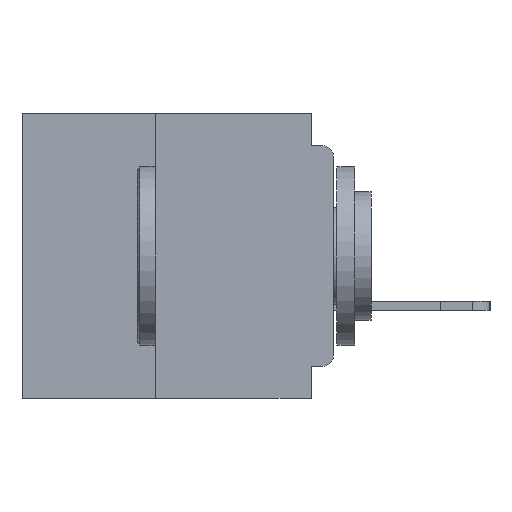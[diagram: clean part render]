
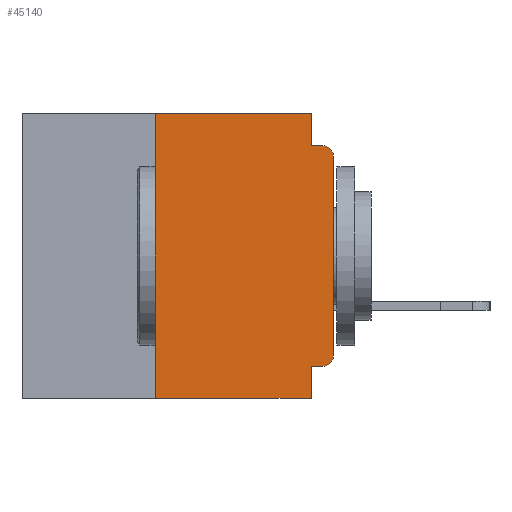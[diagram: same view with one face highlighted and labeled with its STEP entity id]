
A CAD part, left-side view. The second image highlights one B-rep face of the part: STEP entity #45140.
In plain terms, the highlighted planar face has unit normal (-1, 0, 0).
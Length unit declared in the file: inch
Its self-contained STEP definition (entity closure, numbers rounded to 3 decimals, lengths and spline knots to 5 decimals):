
#1364 = VECTOR ( 'NONE', #36220, 39.37008 ) ;
#1433 = VERTEX_POINT ( 'NONE', #27014 ) ;
#1634 = VECTOR ( 'NONE', #19848, 39.37008 ) ;
#1896 = VERTEX_POINT ( 'NONE', #3787 ) ;
#2962 = ORIENTED_EDGE ( 'NONE', *, *, #20656, .T. ) ;
#3313 = VERTEX_POINT ( 'NONE', #28480 ) ;
#3325 = FACE_OUTER_BOUND ( 'NONE', #16595, .T. ) ;
#3534 = DIRECTION ( 'NONE',  ( 0., -1., 0. ) ) ;
#3787 = CARTESIAN_POINT ( 'NONE',  ( 0., 0.031, -0.4 ) ) ;
#5828 = EDGE_CURVE ( 'NONE', #42242, #43689, #36878, .T. ) ;
#5871 = CARTESIAN_POINT ( 'NONE',  ( 0., 0.437, 0. ) ) ;
#6412 = LINE ( 'NONE', #35386, #26719 ) ;
#7238 = CARTESIAN_POINT ( 'NONE',  ( 0., 0.015, -0.06 ) ) ;
#7446 = ORIENTED_EDGE ( 'NONE', *, *, #46930, .F. ) ;
#8452 = AXIS2_PLACEMENT_3D ( 'NONE', #19461, #46099, #23297 ) ;
#9111 = CIRCLE ( 'NONE', #8452, 0.015 ) ;
#9118 = EDGE_CURVE ( 'NONE', #3313, #1896, #33009, .T. ) ;
#9823 = CARTESIAN_POINT ( 'NONE',  ( 0., 0., -0.355 ) ) ;
#10975 = AXIS2_PLACEMENT_3D ( 'NONE', #36495, #21384, #48017 ) ;
#11075 = DIRECTION ( 'NONE',  ( 0., 0., -1. ) ) ;
#12781 = CARTESIAN_POINT ( 'NONE',  ( 0., 0.25, -0.4 ) ) ;
#13275 = ORIENTED_EDGE ( 'NONE', *, *, #5828, .F. ) ;
#14366 = ORIENTED_EDGE ( 'NONE', *, *, #28256, .F. ) ;
#14756 = VERTEX_POINT ( 'NONE', #32859 ) ;
#15012 = CARTESIAN_POINT ( 'NONE',  ( 0., 0.25, 0. ) ) ;
#15478 = ORIENTED_EDGE ( 'NONE', *, *, #43362, .F. ) ;
#16577 = CARTESIAN_POINT ( 'NONE',  ( 0., 0.437, -0.4 ) ) ;
#16595 = EDGE_LOOP ( 'NONE', ( #2962, #45476, #13275, #15478, #44065, #14366, #34073, #23462, #7446, #43950 ) ) ;
#16642 = DIRECTION ( 'NONE',  ( 0., 0., 1. ) ) ;
#17417 = VERTEX_POINT ( 'NONE', #36059 ) ;
#19124 = LINE ( 'NONE', #9823, #39336 ) ;
#19386 = LINE ( 'NONE', #12781, #38417 ) ;
#19461 = CARTESIAN_POINT ( 'NONE',  ( 0., 0.015, -0.34 ) ) ;
#19848 = DIRECTION ( 'NONE',  ( 0., 0., 1. ) ) ;
#20656 = EDGE_CURVE ( 'NONE', #30267, #1433, #42254, .T. ) ;
#21384 = DIRECTION ( 'NONE',  ( 1., 0., 0. ) ) ;
#22906 = CIRCLE ( 'NONE', #28927, 0.015 ) ;
#23297 = DIRECTION ( 'NONE',  ( 0., 0., -1. ) ) ;
#23462 = ORIENTED_EDGE ( 'NONE', *, *, #47915, .F. ) ;
#24372 = VECTOR ( 'NONE', #29343, 39.37008 ) ;
#25028 = PLANE ( 'NONE',  #10975 ) ;
#25037 = DIRECTION ( 'NONE',  ( 0., 1., 0. ) ) ;
#26719 = VECTOR ( 'NONE', #46736, 39.37008 ) ;
#26741 = VECTOR ( 'NONE', #3534, 39.37008 ) ;
#27014 = CARTESIAN_POINT ( 'NONE',  ( 0., 0., -0.06 ) ) ;
#28256 = EDGE_CURVE ( 'NONE', #3313, #44262, #19386, .T. ) ;
#28480 = CARTESIAN_POINT ( 'NONE',  ( 0., 0.25, -0.4 ) ) ;
#28710 = EDGE_CURVE ( 'NONE', #17417, #30267, #9111, .T. ) ;
#28927 = AXIS2_PLACEMENT_3D ( 'NONE', #7238, #33923, #11075 ) ;
#29343 = DIRECTION ( 'NONE',  ( 0., 0., -1. ) ) ;
#29833 = CARTESIAN_POINT ( 'NONE',  ( 0., 0.015, -0.045 ) ) ;
#30267 = VERTEX_POINT ( 'NONE', #33753 ) ;
#31727 = DIRECTION ( 'NONE',  ( 0., -1., 0. ) ) ;
#32859 = CARTESIAN_POINT ( 'NONE',  ( 0., 0.031, -0.355 ) ) ;
#33009 = LINE ( 'NONE', #16577, #44384 ) ;
#33212 = CARTESIAN_POINT ( 'NONE',  ( 0., 0.031, 0. ) ) ;
#33753 = CARTESIAN_POINT ( 'NONE',  ( 0., 0., -0.34 ) ) ;
#33923 = DIRECTION ( 'NONE',  ( -1., 0., 0. ) ) ;
#34073 = ORIENTED_EDGE ( 'NONE', *, *, #9118, .T. ) ;
#35386 = CARTESIAN_POINT ( 'NONE',  ( 0., 0.031, 0. ) ) ;
#36059 = CARTESIAN_POINT ( 'NONE',  ( 0., 0.015, -0.355 ) ) ;
#36220 = DIRECTION ( 'NONE',  ( 0., -1., 0. ) ) ;
#36495 = CARTESIAN_POINT ( 'NONE',  ( 0., 0.437, 0. ) ) ;
#36734 = VERTEX_POINT ( 'NONE', #33212 ) ;
#36878 = LINE ( 'NONE', #49217, #26741 ) ;
#38056 = EDGE_CURVE ( 'NONE', #1433, #43689, #22906, .T. ) ;
#38417 = VECTOR ( 'NONE', #16642, 39.37008 ) ;
#38803 = CARTESIAN_POINT ( 'NONE',  ( 0., 0., 0. ) ) ;
#39336 = VECTOR ( 'NONE', #25037, 39.37008 ) ;
#39982 = CARTESIAN_POINT ( 'NONE',  ( 0., 0.031, -0.045 ) ) ;
#40212 = EDGE_CURVE ( 'NONE', #44262, #36734, #41994, .T. ) ;
#40858 = CARTESIAN_POINT ( 'NONE',  ( 0., 0.031, -0.4 ) ) ;
#41994 = LINE ( 'NONE', #5871, #1364 ) ;
#42242 = VERTEX_POINT ( 'NONE', #39982 ) ;
#42254 = LINE ( 'NONE', #38803, #1634 ) ;
#43362 = EDGE_CURVE ( 'NONE', #36734, #42242, #6412, .T. ) ;
#43689 = VERTEX_POINT ( 'NONE', #29833 ) ;
#43950 = ORIENTED_EDGE ( 'NONE', *, *, #28710, .T. ) ;
#44065 = ORIENTED_EDGE ( 'NONE', *, *, #40212, .F. ) ;
#44262 = VERTEX_POINT ( 'NONE', #15012 ) ;
#44384 = VECTOR ( 'NONE', #31727, 39.37008 ) ;
#45140 = ADVANCED_FACE ( 'NONE', ( #3325 ), #25028, .F. ) ;
#45476 = ORIENTED_EDGE ( 'NONE', *, *, #38056, .T. ) ;
#46099 = DIRECTION ( 'NONE',  ( -1., 0., 0. ) ) ;
#46736 = DIRECTION ( 'NONE',  ( 0., 0., -1. ) ) ;
#46930 = EDGE_CURVE ( 'NONE', #17417, #14756, #19124, .T. ) ;
#47031 = LINE ( 'NONE', #40858, #24372 ) ;
#47915 = EDGE_CURVE ( 'NONE', #14756, #1896, #47031, .T. ) ;
#48017 = DIRECTION ( 'NONE',  ( 0., 0., -1. ) ) ;
#49217 = CARTESIAN_POINT ( 'NONE',  ( 0., 0., -0.045 ) ) ;
